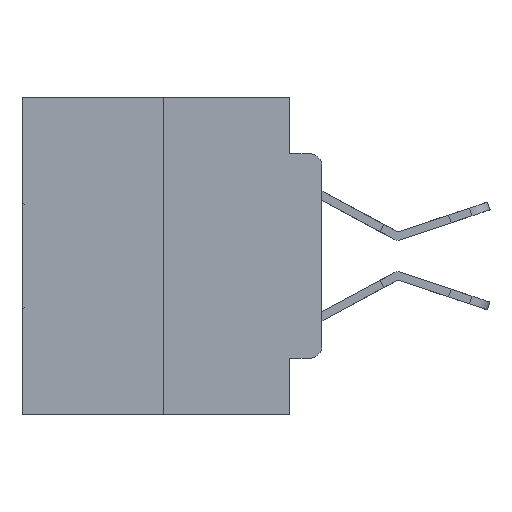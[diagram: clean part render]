
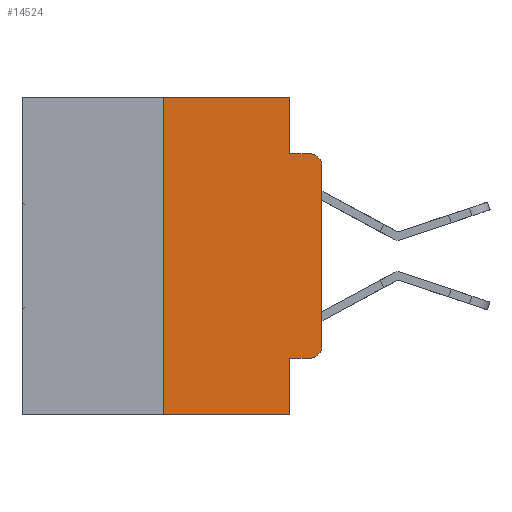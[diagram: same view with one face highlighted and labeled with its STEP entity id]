
A CAD part, left-side view. The second image highlights one B-rep face of the part: STEP entity #14524.
In plain terms, the highlighted planar face has unit normal (-1, 0, 0).
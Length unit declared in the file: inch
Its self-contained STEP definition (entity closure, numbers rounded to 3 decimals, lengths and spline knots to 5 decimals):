
#386 = CARTESIAN_POINT ( 'NONE',  ( 0., 0., 0. ) ) ;
#730 = VERTEX_POINT ( 'NONE', #15926 ) ;
#1260 = DIRECTION ( 'NONE',  ( 0., 0., 1. ) ) ;
#1343 = ORIENTED_EDGE ( 'NONE', *, *, #24738, .T. ) ;
#1515 = VECTOR ( 'NONE', #8685, 39.37008 ) ;
#2492 = EDGE_CURVE ( 'NONE', #29804, #18218, #7850, .T. ) ;
#4039 = VECTOR ( 'NONE', #28094, 39.37008 ) ;
#4806 = ORIENTED_EDGE ( 'NONE', *, *, #21328, .T. ) ;
#6145 = EDGE_CURVE ( 'NONE', #13892, #27046, #9800, .T. ) ;
#6339 = ORIENTED_EDGE ( 'NONE', *, *, #21239, .F. ) ;
#7058 = VERTEX_POINT ( 'NONE', #26054 ) ;
#7514 = VERTEX_POINT ( 'NONE', #20962 ) ;
#7561 = DIRECTION ( 'NONE',  ( 0., -1., 0. ) ) ;
#7596 = PLANE ( 'NONE',  #23107 ) ;
#7850 = LINE ( 'NONE', #12560, #19762 ) ;
#7917 = ORIENTED_EDGE ( 'NONE', *, *, #2492, .F. ) ;
#8154 = CIRCLE ( 'NONE', #26507, 0.02 ) ;
#8685 = DIRECTION ( 'NONE',  ( 0., -1., 0. ) ) ;
#9695 = EDGE_CURVE ( 'NONE', #7058, #730, #25857, .T. ) ;
#9800 = LINE ( 'NONE', #21054, #28667 ) ;
#10303 = FACE_OUTER_BOUND ( 'NONE', #27584, .T. ) ;
#10964 = DIRECTION ( 'NONE',  ( 0., 0., -1. ) ) ;
#11174 = CARTESIAN_POINT ( 'NONE',  ( 0., 0.02, -0.1085 ) ) ;
#12431 = DIRECTION ( 'NONE',  ( 0., 0., -1. ) ) ;
#12560 = CARTESIAN_POINT ( 'NONE',  ( 0., 0.051, 0. ) ) ;
#12697 = CARTESIAN_POINT ( 'NONE',  ( 0., 0.051, 0. ) ) ;
#13473 = DIRECTION ( 'NONE',  ( -1., 0., 0. ) ) ;
#13536 = CARTESIAN_POINT ( 'NONE',  ( 0., 0.473, -0.5 ) ) ;
#13623 = DIRECTION ( 'NONE',  ( 0., 0., -1. ) ) ;
#13892 = VERTEX_POINT ( 'NONE', #14889 ) ;
#13993 = CARTESIAN_POINT ( 'NONE',  ( 0., 0.051, -0.4115 ) ) ;
#14524 = ADVANCED_FACE ( 'NONE', ( #10303 ), #7596, .F. ) ;
#14871 = CARTESIAN_POINT ( 'NONE',  ( 0., 0., -0.1085 ) ) ;
#14889 = CARTESIAN_POINT ( 'NONE',  ( 0., 0.051, -0.0885 ) ) ;
#15785 = ORIENTED_EDGE ( 'NONE', *, *, #29500, .T. ) ;
#15814 = CARTESIAN_POINT ( 'NONE',  ( 0., 0.25, 0. ) ) ;
#15926 = CARTESIAN_POINT ( 'NONE',  ( 0., 0.25, 0. ) ) ;
#16501 = EDGE_CURVE ( 'NONE', #29804, #18255, #22380, .T. ) ;
#16659 = VERTEX_POINT ( 'NONE', #16864 ) ;
#16864 = CARTESIAN_POINT ( 'NONE',  ( 0., 0., -0.3915 ) ) ;
#17363 = DIRECTION ( 'NONE',  ( 0., 0., 1. ) ) ;
#17592 = EDGE_CURVE ( 'NONE', #30185, #27046, #23108, .T. ) ;
#17597 = ORIENTED_EDGE ( 'NONE', *, *, #17592, .T. ) ;
#17646 = CARTESIAN_POINT ( 'NONE',  ( 0., 0.051, -0.4115 ) ) ;
#18218 = VERTEX_POINT ( 'NONE', #30120 ) ;
#18255 = VERTEX_POINT ( 'NONE', #25625 ) ;
#18467 = LINE ( 'NONE', #386, #25472 ) ;
#18880 = VECTOR ( 'NONE', #1260, 39.37008 ) ;
#19762 = VECTOR ( 'NONE', #10964, 39.37008 ) ;
#20720 = LINE ( 'NONE', #13536, #1515 ) ;
#20962 = CARTESIAN_POINT ( 'NONE',  ( 0., 0.051, 0. ) ) ;
#21054 = CARTESIAN_POINT ( 'NONE',  ( 0., 0.051, -0.0885 ) ) ;
#21239 = EDGE_CURVE ( 'NONE', #730, #7514, #26937, .T. ) ;
#21328 = EDGE_CURVE ( 'NONE', #16659, #30185, #18467, .T. ) ;
#21403 = VECTOR ( 'NONE', #7561, 39.37008 ) ;
#21776 = CARTESIAN_POINT ( 'NONE',  ( 0., 0.473, 0. ) ) ;
#22176 = DIRECTION ( 'NONE',  ( 0., 0., -1. ) ) ;
#22380 = LINE ( 'NONE', #13993, #4039 ) ;
#23107 = AXIS2_PLACEMENT_3D ( 'NONE', #24207, #26576, #12431 ) ;
#23108 = CIRCLE ( 'NONE', #25577, 0.02 ) ;
#23139 = EDGE_CURVE ( 'NONE', #7514, #13892, #23877, .T. ) ;
#23877 = LINE ( 'NONE', #12697, #24628 ) ;
#24207 = CARTESIAN_POINT ( 'NONE',  ( 0., 0.473, 0. ) ) ;
#24624 = ORIENTED_EDGE ( 'NONE', *, *, #6145, .F. ) ;
#24628 = VECTOR ( 'NONE', #22176, 39.37008 ) ;
#24738 = EDGE_CURVE ( 'NONE', #7058, #18218, #20720, .T. ) ;
#25472 = VECTOR ( 'NONE', #17363, 39.37008 ) ;
#25577 = AXIS2_PLACEMENT_3D ( 'NONE', #11174, #27729, #13623 ) ;
#25625 = CARTESIAN_POINT ( 'NONE',  ( 0., 0.02, -0.4115 ) ) ;
#25857 = LINE ( 'NONE', #15814, #18880 ) ;
#26054 = CARTESIAN_POINT ( 'NONE',  ( 0., 0.25, -0.5 ) ) ;
#26099 = ORIENTED_EDGE ( 'NONE', *, *, #9695, .F. ) ;
#26507 = AXIS2_PLACEMENT_3D ( 'NONE', #27577, #13473, #29908 ) ;
#26576 = DIRECTION ( 'NONE',  ( 1., 0., 0. ) ) ;
#26937 = LINE ( 'NONE', #21776, #21403 ) ;
#27046 = VERTEX_POINT ( 'NONE', #29638 ) ;
#27570 = ORIENTED_EDGE ( 'NONE', *, *, #16501, .T. ) ;
#27577 = CARTESIAN_POINT ( 'NONE',  ( 0., 0.02, -0.3915 ) ) ;
#27584 = EDGE_LOOP ( 'NONE', ( #4806, #17597, #24624, #30817, #6339, #26099, #1343, #7917, #27570, #15785 ) ) ;
#27729 = DIRECTION ( 'NONE',  ( -1., 0., 0. ) ) ;
#28087 = DIRECTION ( 'NONE',  ( 0., -1., 0. ) ) ;
#28094 = DIRECTION ( 'NONE',  ( 0., -1., 0. ) ) ;
#28667 = VECTOR ( 'NONE', #28087, 39.37008 ) ;
#29500 = EDGE_CURVE ( 'NONE', #18255, #16659, #8154, .T. ) ;
#29638 = CARTESIAN_POINT ( 'NONE',  ( 0., 0.02, -0.0885 ) ) ;
#29804 = VERTEX_POINT ( 'NONE', #17646 ) ;
#29908 = DIRECTION ( 'NONE',  ( 0., 0., -1. ) ) ;
#30120 = CARTESIAN_POINT ( 'NONE',  ( 0., 0.051, -0.5 ) ) ;
#30185 = VERTEX_POINT ( 'NONE', #14871 ) ;
#30817 = ORIENTED_EDGE ( 'NONE', *, *, #23139, .F. ) ;
